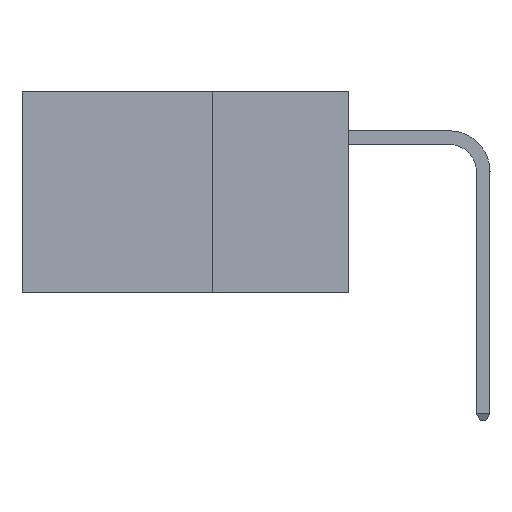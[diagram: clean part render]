
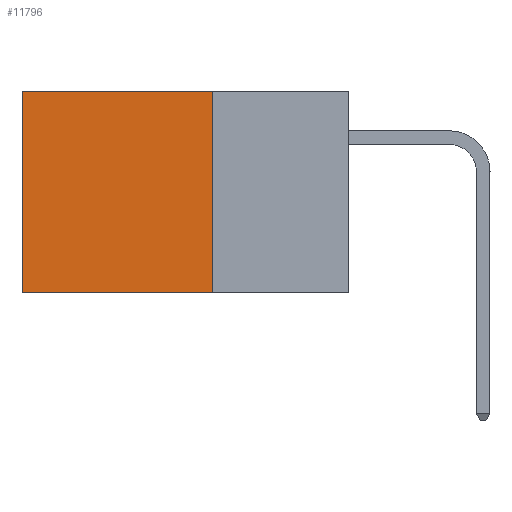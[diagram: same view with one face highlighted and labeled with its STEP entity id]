
A CAD part, left-side view. The second image highlights one B-rep face of the part: STEP entity #11796.
In plain terms, the highlighted planar face has unit normal (-1, 0, 0).
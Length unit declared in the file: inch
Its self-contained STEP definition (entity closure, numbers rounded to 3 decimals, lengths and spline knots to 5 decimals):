
#708 = ORIENTED_EDGE ( 'NONE', *, *, #8961, .F. ) ;
#902 = VECTOR ( 'NONE', #2071, 39.37008 ) ;
#1556 = ORIENTED_EDGE ( 'NONE', *, *, #24031, .T. ) ;
#1977 = VERTEX_POINT ( 'NONE', #18664 ) ;
#2071 = DIRECTION ( 'NONE',  ( 0., 1., 0. ) ) ;
#3339 = EDGE_CURVE ( 'NONE', #4636, #1977, #23664, .T. ) ;
#4636 = VERTEX_POINT ( 'NONE', #13954 ) ;
#5375 = CARTESIAN_POINT ( 'NONE',  ( 0.2875, 0.25, 0. ) ) ;
#5430 = LINE ( 'NONE', #7672, #902 ) ;
#6251 = EDGE_LOOP ( 'NONE', ( #16959, #16475, #708, #1556 ) ) ;
#6321 = VERTEX_POINT ( 'NONE', #21366 ) ;
#6378 = CARTESIAN_POINT ( 'NONE',  ( 0.2875, 0.25, 0. ) ) ;
#6622 = VECTOR ( 'NONE', #17635, 39.37008 ) ;
#7050 = CARTESIAN_POINT ( 'NONE',  ( 0.2875, 0.25, -0.37 ) ) ;
#7672 = CARTESIAN_POINT ( 'NONE',  ( 0.2875, 0.25, 0. ) ) ;
#8243 = LINE ( 'NONE', #5375, #12596 ) ;
#8961 = EDGE_CURVE ( 'NONE', #6321, #9400, #8243, .T. ) ;
#9400 = VERTEX_POINT ( 'NONE', #7050 ) ;
#10098 = CARTESIAN_POINT ( 'NONE',  ( 0.2875, 0.25, -0.37 ) ) ;
#10212 = CARTESIAN_POINT ( 'NONE',  ( 0.2875, 0.6, 0. ) ) ;
#10802 = FACE_OUTER_BOUND ( 'NONE', #6251, .T. ) ;
#11796 = ADVANCED_FACE ( 'NONE', ( #10802 ), #19432, .F. ) ;
#11953 = DIRECTION ( 'NONE',  ( 0., 0., -1. ) ) ;
#12596 = VECTOR ( 'NONE', #20281, 39.37008 ) ;
#13954 = CARTESIAN_POINT ( 'NONE',  ( 0.2875, 0.6, 0. ) ) ;
#15064 = AXIS2_PLACEMENT_3D ( 'NONE', #6378, #23120, #11953 ) ;
#16475 = ORIENTED_EDGE ( 'NONE', *, *, #22437, .F. ) ;
#16535 = LINE ( 'NONE', #10098, #6622 ) ;
#16959 = ORIENTED_EDGE ( 'NONE', *, *, #3339, .T. ) ;
#17635 = DIRECTION ( 'NONE',  ( 0., 1., 0. ) ) ;
#18664 = CARTESIAN_POINT ( 'NONE',  ( 0.2875, 0.6, -0.37 ) ) ;
#19337 = VECTOR ( 'NONE', #21403, 39.37008 ) ;
#19432 = PLANE ( 'NONE',  #15064 ) ;
#20281 = DIRECTION ( 'NONE',  ( 0., 0., -1. ) ) ;
#21366 = CARTESIAN_POINT ( 'NONE',  ( 0.2875, 0.25, 0. ) ) ;
#21403 = DIRECTION ( 'NONE',  ( 0., 0., -1. ) ) ;
#22437 = EDGE_CURVE ( 'NONE', #9400, #1977, #16535, .T. ) ;
#23120 = DIRECTION ( 'NONE',  ( 1., 0., 0. ) ) ;
#23664 = LINE ( 'NONE', #10212, #19337 ) ;
#24031 = EDGE_CURVE ( 'NONE', #6321, #4636, #5430, .T. ) ;
